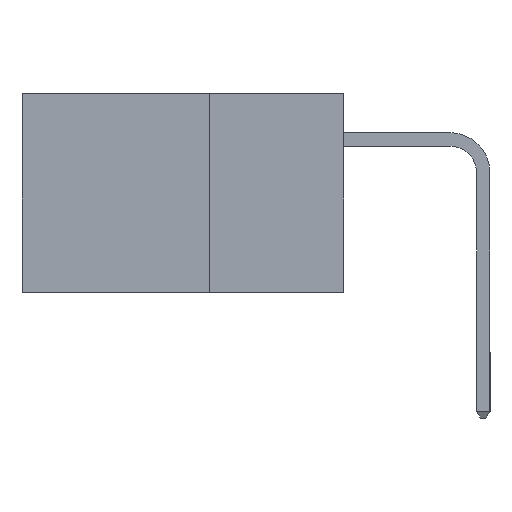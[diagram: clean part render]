
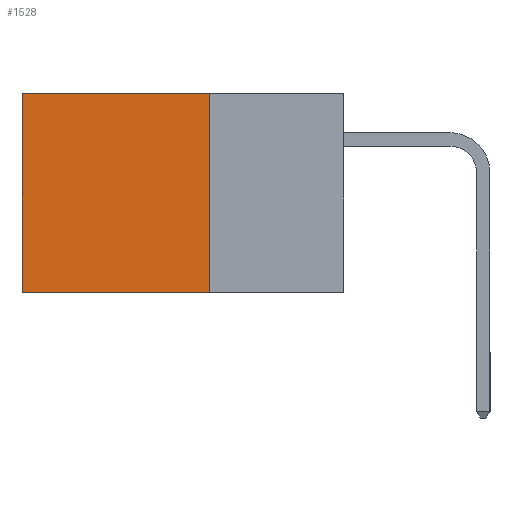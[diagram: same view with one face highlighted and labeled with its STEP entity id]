
A CAD part, left-side view. The second image highlights one B-rep face of the part: STEP entity #1528.
In plain terms, the highlighted planar face has unit normal (-1, 0, 0).
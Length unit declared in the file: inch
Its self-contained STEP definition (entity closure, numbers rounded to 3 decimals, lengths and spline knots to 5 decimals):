
#117 = DIRECTION ( 'NONE',  ( 0., 0., -1. ) ) ;
#269 = CARTESIAN_POINT ( 'NONE',  ( 0.298, 0.25, 0. ) ) ;
#295 = AXIS2_PLACEMENT_3D ( 'NONE', #269, #3862, #5554 ) ;
#329 = LINE ( 'NONE', #7078, #9305 ) ;
#380 = PLANE ( 'NONE',  #295 ) ;
#838 = VERTEX_POINT ( 'NONE', #5980 ) ;
#963 = ORIENTED_EDGE ( 'NONE', *, *, #4522, .F. ) ;
#1087 = VERTEX_POINT ( 'NONE', #9540 ) ;
#1528 = ADVANCED_FACE ( 'NONE', ( #6279 ), #380, .F. ) ;
#1785 = VECTOR ( 'NONE', #117, 39.37008 ) ;
#3351 = VECTOR ( 'NONE', #8308, 39.37008 ) ;
#3356 = VERTEX_POINT ( 'NONE', #9484 ) ;
#3697 = CARTESIAN_POINT ( 'NONE',  ( 0.298, 0.25, 0. ) ) ;
#3862 = DIRECTION ( 'NONE',  ( 1., 0., 0. ) ) ;
#4090 = LINE ( 'NONE', #3697, #1785 ) ;
#4137 = CARTESIAN_POINT ( 'NONE',  ( 0.298, 0.6, 0. ) ) ;
#4179 = LINE ( 'NONE', #4137, #5245 ) ;
#4522 = EDGE_CURVE ( 'NONE', #7984, #838, #4090, .T. ) ;
#4696 = EDGE_CURVE ( 'NONE', #838, #3356, #9309, .T. ) ;
#5082 = DIRECTION ( 'NONE',  ( 0., 0., -1. ) ) ;
#5245 = VECTOR ( 'NONE', #5082, 39.37008 ) ;
#5554 = DIRECTION ( 'NONE',  ( 0., 0., -1. ) ) ;
#5980 = CARTESIAN_POINT ( 'NONE',  ( 0.298, 0.25, -0.37 ) ) ;
#6264 = ORIENTED_EDGE ( 'NONE', *, *, #7555, .T. ) ;
#6279 = FACE_OUTER_BOUND ( 'NONE', #8116, .T. ) ;
#7078 = CARTESIAN_POINT ( 'NONE',  ( 0.298, 0.25, 0. ) ) ;
#7555 = EDGE_CURVE ( 'NONE', #1087, #3356, #4179, .T. ) ;
#7932 = DIRECTION ( 'NONE',  ( 0., 1., 0. ) ) ;
#7984 = VERTEX_POINT ( 'NONE', #8151 ) ;
#8116 = EDGE_LOOP ( 'NONE', ( #6264, #10426, #963, #8585 ) ) ;
#8151 = CARTESIAN_POINT ( 'NONE',  ( 0.298, 0.25, 0. ) ) ;
#8308 = DIRECTION ( 'NONE',  ( 0., 1., 0. ) ) ;
#8585 = ORIENTED_EDGE ( 'NONE', *, *, #10795, .T. ) ;
#9305 = VECTOR ( 'NONE', #7932, 39.37008 ) ;
#9309 = LINE ( 'NONE', #10174, #3351 ) ;
#9484 = CARTESIAN_POINT ( 'NONE',  ( 0.298, 0.6, -0.37 ) ) ;
#9540 = CARTESIAN_POINT ( 'NONE',  ( 0.298, 0.6, 0. ) ) ;
#10174 = CARTESIAN_POINT ( 'NONE',  ( 0.298, 0.25, -0.37 ) ) ;
#10426 = ORIENTED_EDGE ( 'NONE', *, *, #4696, .F. ) ;
#10795 = EDGE_CURVE ( 'NONE', #7984, #1087, #329, .T. ) ;
